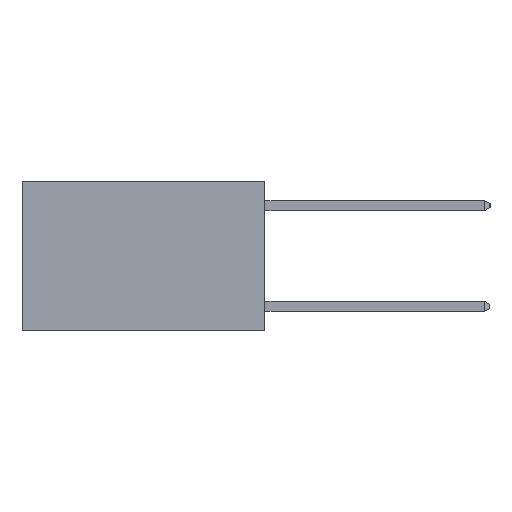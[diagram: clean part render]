
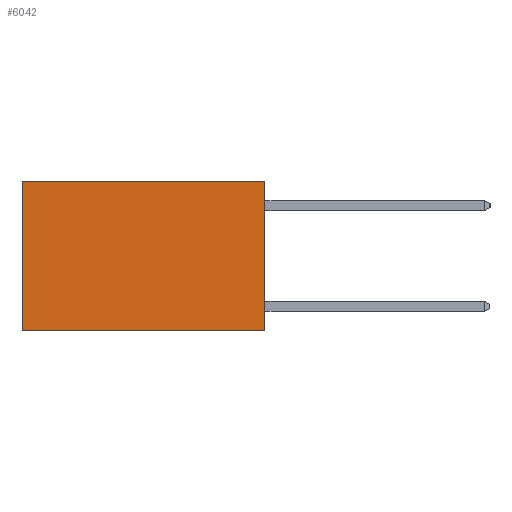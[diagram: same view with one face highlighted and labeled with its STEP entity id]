
A CAD part, left-side view. The second image highlights one B-rep face of the part: STEP entity #6042.
In plain terms, the highlighted planar face has unit normal (-1, 0, 0).
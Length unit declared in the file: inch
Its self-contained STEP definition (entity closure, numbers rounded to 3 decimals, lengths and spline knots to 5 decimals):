
#311 = CARTESIAN_POINT ( 'NONE',  ( 0.2625, 0.6, 0. ) ) ;
#423 = EDGE_CURVE ( 'NONE', #773, #4163, #3918, .T. ) ;
#634 = EDGE_CURVE ( 'NONE', #1326, #3455, #4569, .T. ) ;
#773 = VERTEX_POINT ( 'NONE', #3671 ) ;
#889 = CARTESIAN_POINT ( 'NONE',  ( 0.2625, 0., 0. ) ) ;
#933 = AXIS2_PLACEMENT_3D ( 'NONE', #2461, #8313, #3343 ) ;
#1326 = VERTEX_POINT ( 'NONE', #5104 ) ;
#1629 = VECTOR ( 'NONE', #3211, 39.37008 ) ;
#1643 = VECTOR ( 'NONE', #4352, 39.37008 ) ;
#1742 = EDGE_CURVE ( 'NONE', #1326, #773, #10445, .T. ) ;
#2269 = ORIENTED_EDGE ( 'NONE', *, *, #5783, .T. ) ;
#2461 = CARTESIAN_POINT ( 'NONE',  ( 0.2625, 0., 0. ) ) ;
#2660 = CARTESIAN_POINT ( 'NONE',  ( 0.2625, 0.6, 0. ) ) ;
#3211 = DIRECTION ( 'NONE',  ( 0., 1., 0. ) ) ;
#3343 = DIRECTION ( 'NONE',  ( 0., 0., -1. ) ) ;
#3455 = VERTEX_POINT ( 'NONE', #2660 ) ;
#3618 = ORIENTED_EDGE ( 'NONE', *, *, #423, .F. ) ;
#3671 = CARTESIAN_POINT ( 'NONE',  ( 0.2625, 0., -0.37 ) ) ;
#3819 = ORIENTED_EDGE ( 'NONE', *, *, #634, .T. ) ;
#3918 = LINE ( 'NONE', #6627, #1629 ) ;
#4163 = VERTEX_POINT ( 'NONE', #7765 ) ;
#4352 = DIRECTION ( 'NONE',  ( 0., 0., -1. ) ) ;
#4375 = FACE_OUTER_BOUND ( 'NONE', #9926, .T. ) ;
#4569 = LINE ( 'NONE', #8110, #8444 ) ;
#5104 = CARTESIAN_POINT ( 'NONE',  ( 0.2625, 0., 0. ) ) ;
#5310 = VECTOR ( 'NONE', #5491, 39.37008 ) ;
#5491 = DIRECTION ( 'NONE',  ( 0., 0., -1. ) ) ;
#5783 = EDGE_CURVE ( 'NONE', #3455, #4163, #9640, .T. ) ;
#5861 = PLANE ( 'NONE',  #933 ) ;
#6042 = ADVANCED_FACE ( 'NONE', ( #4375 ), #5861, .F. ) ;
#6627 = CARTESIAN_POINT ( 'NONE',  ( 0.2625, 0., -0.37 ) ) ;
#7635 = DIRECTION ( 'NONE',  ( 0., 1., 0. ) ) ;
#7765 = CARTESIAN_POINT ( 'NONE',  ( 0.2625, 0.6, -0.37 ) ) ;
#8110 = CARTESIAN_POINT ( 'NONE',  ( 0.2625, 0., 0. ) ) ;
#8313 = DIRECTION ( 'NONE',  ( 1., 0., 0. ) ) ;
#8444 = VECTOR ( 'NONE', #7635, 39.37008 ) ;
#8714 = ORIENTED_EDGE ( 'NONE', *, *, #1742, .F. ) ;
#9640 = LINE ( 'NONE', #311, #5310 ) ;
#9926 = EDGE_LOOP ( 'NONE', ( #2269, #3618, #8714, #3819 ) ) ;
#10445 = LINE ( 'NONE', #889, #1643 ) ;
